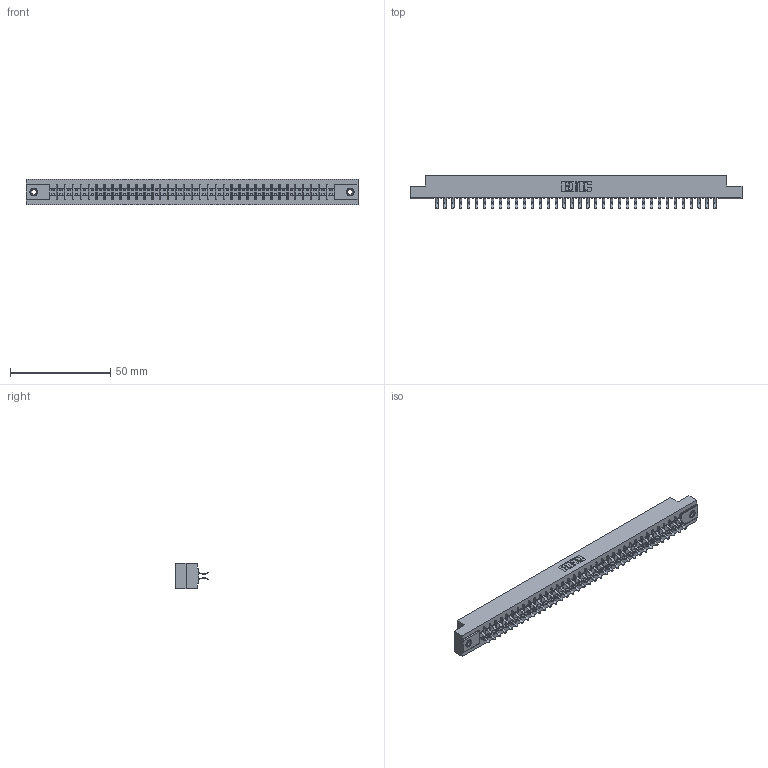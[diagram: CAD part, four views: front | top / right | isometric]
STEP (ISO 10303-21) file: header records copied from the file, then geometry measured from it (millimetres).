
FILE_DESCRIPTION (( 'STEP AP203' ), '1' );
FILE_NAME ('315-072-556-208.STEP', '2019-09-10T21:56:55', ( '' ), ( '' ), 'SwSTEP 2.0', 'SolidWorks 2016', '' );
FILE_SCHEMA (( 'CONFIG_CONTROL_DESIGN' ));
Length unit declared in the file: inch
Products named in the file (4): 315-072-556-208; 305-290-001_556; 305 Part_.156 Dia; 345-250-001_345-250-003-102
Assembly tree (75 placements, depth 2):
  315-072-556-208
    305 Part_.156 Dia
    305-290-001_556  x72
    345-250-001_345-250-003-102  x2
Bounding box: 165.66 x 16.64 x 12.7 mm (x, y, z)
Volume: 17231.3 mm3; surface area: 21823.1 mm2
Topology: 75 solids, 75 shells, 4208 faces, 12080 edges, 7852 vertices
Faces by surface type: plane 2332, cylinder 1716, sphere 144, cone 12, torus 4
Entity records: 41116 total; most frequent: CARTESIAN_POINT 6789, ORIENTED_EDGE 6732, DIRECTION 6586, EDGE_CURVE 3366, LINE 2708, VECTOR 2708, VERTEX_POINT 2142, AXIS2_PLACEMENT_3D 1939
